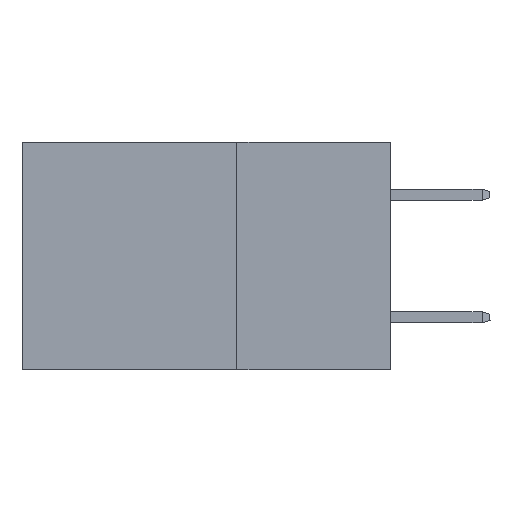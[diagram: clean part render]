
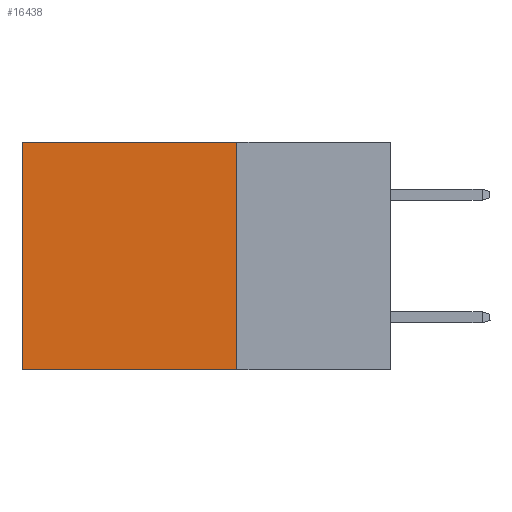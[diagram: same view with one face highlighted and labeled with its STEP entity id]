
A CAD part, left-side view. The second image highlights one B-rep face of the part: STEP entity #16438.
In plain terms, the highlighted planar face has unit normal (-1, 0, 0).
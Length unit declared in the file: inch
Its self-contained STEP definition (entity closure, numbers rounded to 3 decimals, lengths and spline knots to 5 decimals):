
#384 = VECTOR ( 'NONE', #4709, 39.37008 ) ;
#864 = LINE ( 'NONE', #17977, #5364 ) ;
#2033 = VECTOR ( 'NONE', #11888, 39.37008 ) ;
#4709 = DIRECTION ( 'NONE',  ( 0., 0., -1. ) ) ;
#5066 = DIRECTION ( 'NONE',  ( 0., 0., -1. ) ) ;
#5197 = EDGE_CURVE ( 'NONE', #17881, #19939, #864, .T. ) ;
#5364 = VECTOR ( 'NONE', #9807, 39.37008 ) ;
#6912 = CARTESIAN_POINT ( 'NONE',  ( 0.2875, 0.25, 0. ) ) ;
#6985 = EDGE_CURVE ( 'NONE', #17739, #15091, #21516, .T. ) ;
#7421 = ORIENTED_EDGE ( 'NONE', *, *, #5197, .F. ) ;
#8107 = EDGE_CURVE ( 'NONE', #15091, #19939, #10306, .T. ) ;
#8419 = ORIENTED_EDGE ( 'NONE', *, *, #8107, .T. ) ;
#8574 = VECTOR ( 'NONE', #10008, 39.37008 ) ;
#9807 = DIRECTION ( 'NONE',  ( 0., 1., 0. ) ) ;
#10003 = CARTESIAN_POINT ( 'NONE',  ( 0.2875, 0.25, 0. ) ) ;
#10008 = DIRECTION ( 'NONE',  ( 0., 0., -1. ) ) ;
#10306 = LINE ( 'NONE', #14892, #384 ) ;
#10311 = FACE_OUTER_BOUND ( 'NONE', #25788, .T. ) ;
#10713 = CARTESIAN_POINT ( 'NONE',  ( 0.2875, 0.6, -0.37 ) ) ;
#10844 = ORIENTED_EDGE ( 'NONE', *, *, #18760, .F. ) ;
#11888 = DIRECTION ( 'NONE',  ( 0., 1., 0. ) ) ;
#13391 = LINE ( 'NONE', #22217, #8574 ) ;
#14788 = CARTESIAN_POINT ( 'NONE',  ( 0.2875, 0.6, 0. ) ) ;
#14892 = CARTESIAN_POINT ( 'NONE',  ( 0.2875, 0.6, 0. ) ) ;
#15091 = VERTEX_POINT ( 'NONE', #14788 ) ;
#16438 = ADVANCED_FACE ( 'NONE', ( #10311 ), #17300, .F. ) ;
#17300 = PLANE ( 'NONE',  #17612 ) ;
#17612 = AXIS2_PLACEMENT_3D ( 'NONE', #6912, #21204, #5066 ) ;
#17739 = VERTEX_POINT ( 'NONE', #20048 ) ;
#17881 = VERTEX_POINT ( 'NONE', #18558 ) ;
#17977 = CARTESIAN_POINT ( 'NONE',  ( 0.2875, 0.25, -0.37 ) ) ;
#18558 = CARTESIAN_POINT ( 'NONE',  ( 0.2875, 0.25, -0.37 ) ) ;
#18760 = EDGE_CURVE ( 'NONE', #17739, #17881, #13391, .T. ) ;
#19939 = VERTEX_POINT ( 'NONE', #10713 ) ;
#20048 = CARTESIAN_POINT ( 'NONE',  ( 0.2875, 0.25, 0. ) ) ;
#21204 = DIRECTION ( 'NONE',  ( 1., 0., 0. ) ) ;
#21516 = LINE ( 'NONE', #10003, #2033 ) ;
#22217 = CARTESIAN_POINT ( 'NONE',  ( 0.2875, 0.25, 0. ) ) ;
#25606 = ORIENTED_EDGE ( 'NONE', *, *, #6985, .T. ) ;
#25788 = EDGE_LOOP ( 'NONE', ( #8419, #7421, #10844, #25606 ) ) ;
